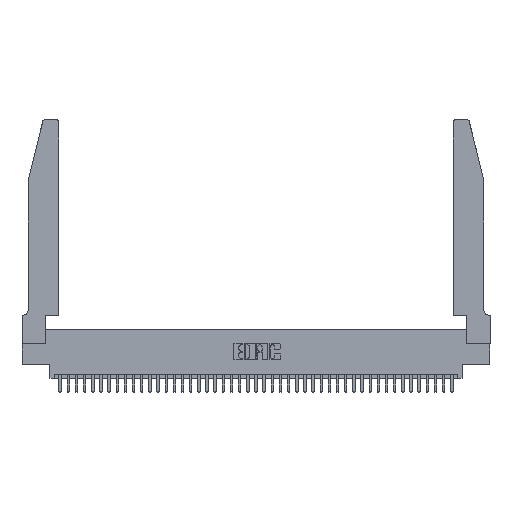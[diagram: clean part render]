
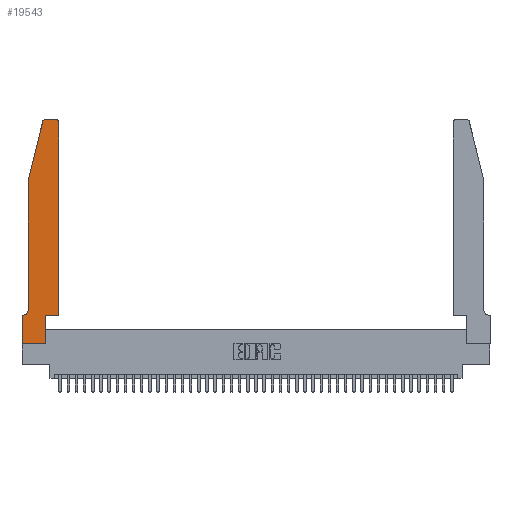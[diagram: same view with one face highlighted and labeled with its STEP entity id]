
A CAD part, top view. The second image highlights one B-rep face of the part: STEP entity #19543.
In plain terms, the highlighted planar face has unit normal (0, 0, 1).
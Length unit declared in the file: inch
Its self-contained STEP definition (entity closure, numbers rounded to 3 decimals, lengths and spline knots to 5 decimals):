
#480 = LINE ( 'NONE', #38086, #15933 ) ;
#637 = EDGE_CURVE ( 'NONE', #20609, #16663, #20458, .T. ) ;
#824 = CARTESIAN_POINT ( 'NONE',  ( 0.4505, 0.35, 0.37 ) ) ;
#1087 = LINE ( 'NONE', #9686, #15487 ) ;
#1163 = VERTEX_POINT ( 'NONE', #3840 ) ;
#1254 = DIRECTION ( 'NONE',  ( 0., 0., -1. ) ) ;
#1312 = VERTEX_POINT ( 'NONE', #20045 ) ;
#1786 = VERTEX_POINT ( 'NONE', #40384 ) ;
#2130 = VERTEX_POINT ( 'NONE', #41463 ) ;
#2383 = ORIENTED_EDGE ( 'NONE', *, *, #8783, .T. ) ;
#2578 = LINE ( 'NONE', #35284, #18521 ) ;
#2689 = VERTEX_POINT ( 'NONE', #4613 ) ;
#2752 = ORIENTED_EDGE ( 'NONE', *, *, #3328, .T. ) ;
#3161 = AXIS2_PLACEMENT_3D ( 'NONE', #34653, #14997, #40441 ) ;
#3277 = VERTEX_POINT ( 'NONE', #22486 ) ;
#3328 = EDGE_CURVE ( 'NONE', #10544, #2130, #27360, .T. ) ;
#3840 = CARTESIAN_POINT ( 'NONE',  ( 0.25487, 2.72718, 0.37 ) ) ;
#4012 = EDGE_CURVE ( 'NONE', #2130, #20609, #480, .T. ) ;
#4287 = AXIS2_PLACEMENT_3D ( 'NONE', #28189, #11791, #38056 ) ;
#4613 = CARTESIAN_POINT ( 'NONE',  ( 0.0755, 2., 0.37 ) ) ;
#4781 = VERTEX_POINT ( 'NONE', #23616 ) ;
#5001 = ORIENTED_EDGE ( 'NONE', *, *, #29989, .T. ) ;
#6408 = ORIENTED_EDGE ( 'NONE', *, *, #34974, .T. ) ;
#7209 = DIRECTION ( 'NONE',  ( 0., -1., 0. ) ) ;
#7335 = DIRECTION ( 'NONE',  ( 1., 0., 0. ) ) ;
#7563 = CARTESIAN_POINT ( 'NONE',  ( 0., 0.35, 0.37 ) ) ;
#7586 = VECTOR ( 'NONE', #10472, 39.37008 ) ;
#7803 = VECTOR ( 'NONE', #7209, 39.37008 ) ;
#8605 = LINE ( 'NONE', #14212, #7586 ) ;
#8783 = EDGE_CURVE ( 'NONE', #33588, #1312, #39057, .T. ) ;
#9686 = CARTESIAN_POINT ( 'NONE',  ( 0.0755, 2., 0.37 ) ) ;
#9849 = AXIS2_PLACEMENT_3D ( 'NONE', #13220, #26194, #22852 ) ;
#10018 = EDGE_CURVE ( 'NONE', #2689, #1786, #8605, .T. ) ;
#10435 = VERTEX_POINT ( 'NONE', #30406 ) ;
#10472 = DIRECTION ( 'NONE',  ( 0., -1., 0. ) ) ;
#10544 = VERTEX_POINT ( 'NONE', #7563 ) ;
#11586 = VECTOR ( 'NONE', #7335, 39.37008 ) ;
#11791 = DIRECTION ( 'NONE',  ( 0., 0., 1. ) ) ;
#12403 = LINE ( 'NONE', #41148, #42210 ) ;
#12878 = EDGE_CURVE ( 'NONE', #1312, #4781, #24805, .T. ) ;
#13148 = AXIS2_PLACEMENT_3D ( 'NONE', #27154, #1254, #17932 ) ;
#13220 = CARTESIAN_POINT ( 'NONE',  ( 0.284, 2.72, 0.37 ) ) ;
#13414 = EDGE_CURVE ( 'NONE', #3277, #33588, #12403, .T. ) ;
#14133 = PLANE ( 'NONE',  #3161 ) ;
#14212 = CARTESIAN_POINT ( 'NONE',  ( 0.0755, 2., 0.37 ) ) ;
#14997 = DIRECTION ( 'NONE',  ( 0., 0., 1. ) ) ;
#15487 = VECTOR ( 'NONE', #32319, 39.37008 ) ;
#15849 = VECTOR ( 'NONE', #25294, 39.37008 ) ;
#15933 = VECTOR ( 'NONE', #28073, 39.37008 ) ;
#16663 = VERTEX_POINT ( 'NONE', #31118 ) ;
#17932 = DIRECTION ( 'NONE',  ( -1., 0., 0. ) ) ;
#18521 = VECTOR ( 'NONE', #29370, 39.37008 ) ;
#18860 = EDGE_CURVE ( 'NONE', #16663, #3277, #20300, .T. ) ;
#18879 = CARTESIAN_POINT ( 'NONE',  ( 0.2605, 2.75, 0.37 ) ) ;
#19306 = ORIENTED_EDGE ( 'NONE', *, *, #10018, .T. ) ;
#19543 = ADVANCED_FACE ( 'NONE', ( #24890 ), #14133, .T. ) ;
#20045 = CARTESIAN_POINT ( 'NONE',  ( 0.4205, 2.75, 0.37 ) ) ;
#20300 = LINE ( 'NONE', #824, #11586 ) ;
#20331 = ORIENTED_EDGE ( 'NONE', *, *, #637, .T. ) ;
#20458 = LINE ( 'NONE', #24853, #15849 ) ;
#20609 = VERTEX_POINT ( 'NONE', #27122 ) ;
#20877 = EDGE_CURVE ( 'NONE', #10435, #10544, #2578, .T. ) ;
#22069 = EDGE_LOOP ( 'NONE', ( #35037, #6408, #5001, #19306, #30557, #38015, #2752, #23211, #20331, #34882, #39200, #2383 ) ) ;
#22486 = CARTESIAN_POINT ( 'NONE',  ( 0.4505, 0.35, 0.37 ) ) ;
#22852 = DIRECTION ( 'NONE',  ( 1., 0., 0. ) ) ;
#23211 = ORIENTED_EDGE ( 'NONE', *, *, #4012, .T. ) ;
#23426 = CARTESIAN_POINT ( 'NONE',  ( 0., 0., 0.37 ) ) ;
#23616 = CARTESIAN_POINT ( 'NONE',  ( 0.284, 2.75, 0.37 ) ) ;
#24805 = LINE ( 'NONE', #18879, #28414 ) ;
#24853 = CARTESIAN_POINT ( 'NONE',  ( 0.2865, 0.35, 0.37 ) ) ;
#24890 = FACE_OUTER_BOUND ( 'NONE', #22069, .T. ) ;
#25294 = DIRECTION ( 'NONE',  ( 0., 1., 0. ) ) ;
#26194 = DIRECTION ( 'NONE',  ( 0., 0., 1. ) ) ;
#27122 = CARTESIAN_POINT ( 'NONE',  ( 0.2865, 0., 0.37 ) ) ;
#27154 = CARTESIAN_POINT ( 'NONE',  ( 0.0055, 0.42, 0.37 ) ) ;
#27360 = LINE ( 'NONE', #23426, #7803 ) ;
#28073 = DIRECTION ( 'NONE',  ( 1., 0., 0. ) ) ;
#28189 = CARTESIAN_POINT ( 'NONE',  ( 0.4205, 2.72, 0.37 ) ) ;
#28414 = VECTOR ( 'NONE', #38825, 39.37008 ) ;
#29370 = DIRECTION ( 'NONE',  ( -1., 0., 0. ) ) ;
#29989 = EDGE_CURVE ( 'NONE', #1163, #2689, #1087, .T. ) ;
#30406 = CARTESIAN_POINT ( 'NONE',  ( 0.0055, 0.35, 0.37 ) ) ;
#30557 = ORIENTED_EDGE ( 'NONE', *, *, #36169, .T. ) ;
#31118 = CARTESIAN_POINT ( 'NONE',  ( 0.2865, 0.35, 0.37 ) ) ;
#32319 = DIRECTION ( 'NONE',  ( -0.239, -0.971, 0. ) ) ;
#33588 = VERTEX_POINT ( 'NONE', #39049 ) ;
#34653 = CARTESIAN_POINT ( 'NONE',  ( 0., 0.35, 0.37 ) ) ;
#34882 = ORIENTED_EDGE ( 'NONE', *, *, #18860, .T. ) ;
#34974 = EDGE_CURVE ( 'NONE', #4781, #1163, #36300, .T. ) ;
#35037 = ORIENTED_EDGE ( 'NONE', *, *, #12878, .T. ) ;
#35246 = CIRCLE ( 'NONE', #13148, 0.07 ) ;
#35284 = CARTESIAN_POINT ( 'NONE',  ( 0.0755, 0.35, 0.37 ) ) ;
#36169 = EDGE_CURVE ( 'NONE', #1786, #10435, #35246, .T. ) ;
#36300 = CIRCLE ( 'NONE', #9849, 0.03 ) ;
#37810 = DIRECTION ( 'NONE',  ( 0., 1., 0. ) ) ;
#38015 = ORIENTED_EDGE ( 'NONE', *, *, #20877, .T. ) ;
#38056 = DIRECTION ( 'NONE',  ( 1., 0., 0. ) ) ;
#38086 = CARTESIAN_POINT ( 'NONE',  ( 0., 0., 0.37 ) ) ;
#38825 = DIRECTION ( 'NONE',  ( -1., 0., 0. ) ) ;
#39049 = CARTESIAN_POINT ( 'NONE',  ( 0.4505, 2.72, 0.37 ) ) ;
#39057 = CIRCLE ( 'NONE', #4287, 0.03 ) ;
#39200 = ORIENTED_EDGE ( 'NONE', *, *, #13414, .T. ) ;
#40384 = CARTESIAN_POINT ( 'NONE',  ( 0.0755, 0.42, 0.37 ) ) ;
#40441 = DIRECTION ( 'NONE',  ( 1., 0., 0. ) ) ;
#41148 = CARTESIAN_POINT ( 'NONE',  ( 0.4505, 0.35, 0.37 ) ) ;
#41463 = CARTESIAN_POINT ( 'NONE',  ( 0., 0., 0.37 ) ) ;
#42210 = VECTOR ( 'NONE', #37810, 39.37008 ) ;
